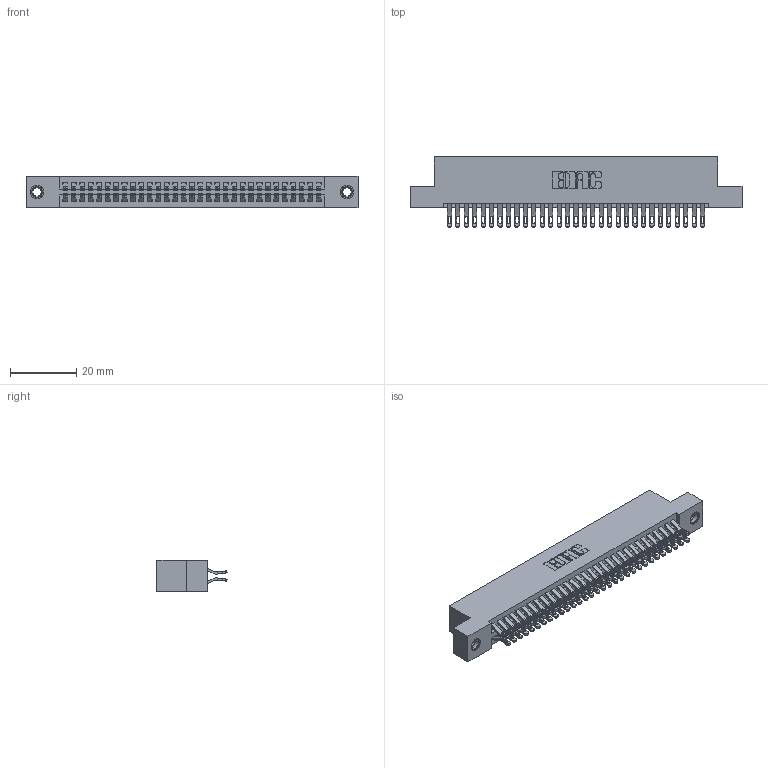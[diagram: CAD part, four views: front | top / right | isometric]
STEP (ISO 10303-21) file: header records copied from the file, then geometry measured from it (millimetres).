
FILE_DESCRIPTION (( 'STEP AP203' ), '1' );
FILE_NAME ('395-062-555-207.STEP', '2018-11-24T04:49:22', ( '' ), ( '' ), 'SwSTEP 2.0', 'SolidWorks 2016', '' );
FILE_SCHEMA (( 'CONFIG_CONTROL_DESIGN' ));
Length unit declared in the file: inch
Products named in the file (4): 395-062-555-207; 345-250-001_345-250-005-103; 345-292-001_555 Tail; 345 Part_Flush Mounting Lugs - 0.156 Dia-TI
Assembly tree (65 placements, depth 2):
  395-062-555-207
    345 Part_Flush Mounting Lugs - 0.156 Dia-TI
    345-292-001_555 Tail  x62
    345-250-001_345-250-005-103  x2
Bounding box: 99.95 x 21.13 x 9.4 mm (x, y, z)
Volume: 9773.4 mm3; surface area: 14887 mm2
Topology: 65 solids, 65 shells, 3658 faces, 11451 edges, 7626 vertices
Faces by surface type: plane 2034, cylinder 1608, cone 12, torus 4
Entity records: 27316 total; most frequent: CARTESIAN_POINT 4605, ORIENTED_EDGE 4502, DIRECTION 4069, EDGE_CURVE 2251, VECTOR 1955, LINE 1955, VERTEX_POINT 1496, AXIS2_PLACEMENT_3D 1057
